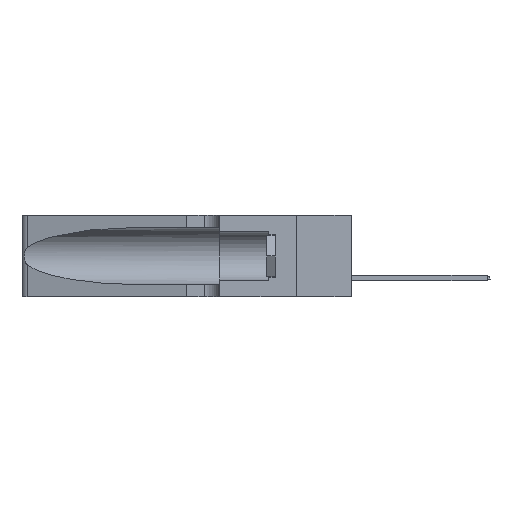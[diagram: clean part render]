
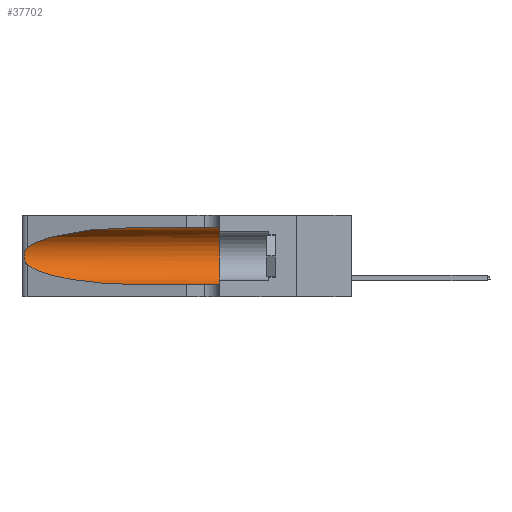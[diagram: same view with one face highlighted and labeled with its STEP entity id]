
A CAD part, left-side view. The second image highlights one B-rep face of the part: STEP entity #37702.
In plain terms, the highlighted cylindrical face has radius 3.308 mm (diameter 6.617 mm), a partial arc.
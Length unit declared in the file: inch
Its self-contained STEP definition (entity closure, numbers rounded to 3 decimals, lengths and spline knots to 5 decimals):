
#49 = EDGE_CURVE ( 'NONE', #26094, #20055, #33524, .T. ) ;
#1766 = ORIENTED_EDGE ( 'NONE', *, *, #3225, .T. ) ;
#2124 =( BOUNDED_CURVE ( )  B_SPLINE_CURVE ( 3, ( #13267, #25940, #29987, #39551 ),
 .UNSPECIFIED., .F., .F. ) 
 B_SPLINE_CURVE_WITH_KNOTS ( ( 4, 4 ),
 ( 3.44316, 4.71239 ),
 .UNSPECIFIED. ) 
 CURVE ( )  GEOMETRIC_REPRESENTATION_ITEM ( )  RATIONAL_B_SPLINE_CURVE ( ( 1., 0.87, 0.87, 1. ) ) 
 REPRESENTATION_ITEM ( '' )  );
#2389 = CARTESIAN_POINT ( 'NONE',  ( 0.26018, 1.23835, 0.19895 ) ) ;
#2554 = ORIENTED_EDGE ( 'NONE', *, *, #24998, .T. ) ;
#2798 = CARTESIAN_POINT ( 'NONE',  ( 0.25789, 1.23486, 0.15765 ) ) ;
#2854 = VECTOR ( 'NONE', #5763, 39.37008 ) ;
#3225 = EDGE_CURVE ( 'NONE', #15961, #3740, #2124, .T. ) ;
#3517 = AXIS2_PLACEMENT_3D ( 'NONE', #11135, #17967, #21017 ) ;
#3740 = VERTEX_POINT ( 'NONE', #24956 ) ;
#3848 = ORIENTED_EDGE ( 'NONE', *, *, #4998, .T. ) ;
#3862 = LINE ( 'NONE', #28295, #2854 ) ;
#4002 = CARTESIAN_POINT ( 'NONE',  ( 0.1305, 0.35, 0.05475 ) ) ;
#4131 = CYLINDRICAL_SURFACE ( 'NONE', #8900, 0.13025 ) ;
#4998 = EDGE_CURVE ( 'NONE', #3740, #20055, #3862, .T. ) ;
#5478 = CARTESIAN_POINT ( 'NONE',  ( 0.25787, 1.23484, 0.2124 ) ) ;
#5595 = CARTESIAN_POINT ( 'NONE',  ( 0.26075, 1.23896, 0.19203 ) ) ;
#5763 = DIRECTION ( 'NONE',  ( 0., -1., 0. ) ) ;
#6062 = DIRECTION ( 'NONE',  ( 0., -1., 0. ) ) ;
#8669 = CARTESIAN_POINT ( 'NONE',  ( 0.1305, 0.35, 0.31525 ) ) ;
#8900 = AXIS2_PLACEMENT_3D ( 'NONE', #13526, #38990, #19927 ) ;
#11135 = CARTESIAN_POINT ( 'NONE',  ( 0.1305, 0.35, 0.185 ) ) ;
#12410 = CARTESIAN_POINT ( 'NONE',  ( 0.25487, 1.22718, 0.22369 ) ) ;
#12671 = LINE ( 'NONE', #37898, #26615 ) ;
#13267 = CARTESIAN_POINT ( 'NONE',  ( 0.25487, 1.22718, 0.14631 ) ) ;
#13526 = CARTESIAN_POINT ( 'NONE',  ( 0.1305, 1.61858, 0.185 ) ) ;
#14025 = CARTESIAN_POINT ( 'NONE',  ( 0.2373, 1.15595, 0.28018 ) ) ;
#14151 = CARTESIAN_POINT ( 'NONE',  ( 0.1305, 0.72297, 0.31525 ) ) ;
#14511 = EDGE_CURVE ( 'NONE', #38973, #26094, #12671, .T. ) ;
#14899 = CARTESIAN_POINT ( 'NONE',  ( 0.25854, 1.2359, 0.20912 ) ) ;
#15696 = CARTESIAN_POINT ( 'NONE',  ( 0.25856, 1.23593, 0.16098 ) ) ;
#15961 = VERTEX_POINT ( 'NONE', #18734 ) ;
#17967 = DIRECTION ( 'NONE',  ( 0., 1., 0. ) ) ;
#18384 = CARTESIAN_POINT ( 'NONE',  ( 0.25555, 1.22994, 0.2215 ) ) ;
#18734 = CARTESIAN_POINT ( 'NONE',  ( 0.25487, 1.22718, 0.14631 ) ) ;
#19927 = DIRECTION ( 'NONE',  ( 0., 0., -1. ) ) ;
#20055 = VERTEX_POINT ( 'NONE', #4002 ) ;
#21017 = DIRECTION ( 'NONE',  ( 0., 0., 1. ) ) ;
#22402 = CARTESIAN_POINT ( 'NONE',  ( 0.25639, 1.23186, 0.15144 ) ) ;
#24956 = CARTESIAN_POINT ( 'NONE',  ( 0.1305, 0.72297, 0.05475 ) ) ;
#24998 = EDGE_CURVE ( 'NONE', #38973, #35078, #38556, .T. ) ;
#25572 = CARTESIAN_POINT ( 'NONE',  ( 0.25555, 1.22993, 0.14849 ) ) ;
#25646 = EDGE_LOOP ( 'NONE', ( #2554, #28320, #1766, #3848, #26276, #35158 ) ) ;
#25940 = CARTESIAN_POINT ( 'NONE',  ( 0.2373, 1.15595, 0.08982 ) ) ;
#26094 = VERTEX_POINT ( 'NONE', #8669 ) ;
#26276 = ORIENTED_EDGE ( 'NONE', *, *, #49, .F. ) ;
#26615 = VECTOR ( 'NONE', #6062, 39.37008 ) ;
#26858 = B_SPLINE_CURVE_WITH_KNOTS ( 'NONE', 3,
 ( #30785, #18384, #33970, #5478, #14899, #2389, #5595, #34247, #40623, #15696, #2798, #22402, #25572, #37967 ),
 .UNSPECIFIED., .F., .F.,
 ( 4, 2, 2, 2, 2, 2, 4 ),
 ( 0., 0.00027, 0.00053, 0.00107, 0.0016, 0.00187, 0.00214 ),
 .UNSPECIFIED. ) ;
#28295 = CARTESIAN_POINT ( 'NONE',  ( 0.1305, 1.61858, 0.05475 ) ) ;
#28320 = ORIENTED_EDGE ( 'NONE', *, *, #39826, .T. ) ;
#29987 = CARTESIAN_POINT ( 'NONE',  ( 0.18966, 0.96281, 0.05475 ) ) ;
#30785 = CARTESIAN_POINT ( 'NONE',  ( 0.25487, 1.22718, 0.22369 ) ) ;
#33469 = CARTESIAN_POINT ( 'NONE',  ( 0.1305, 0.72297, 0.31525 ) ) ;
#33509 = CARTESIAN_POINT ( 'NONE',  ( 0.25487, 1.22718, 0.22369 ) ) ;
#33524 = CIRCLE ( 'NONE', #3517, 0.13025 ) ;
#33970 = CARTESIAN_POINT ( 'NONE',  ( 0.25639, 1.23184, 0.21858 ) ) ;
#34247 = CARTESIAN_POINT ( 'NONE',  ( 0.26075, 1.23896, 0.178 ) ) ;
#35078 = VERTEX_POINT ( 'NONE', #12410 ) ;
#35158 = ORIENTED_EDGE ( 'NONE', *, *, #14511, .F. ) ;
#36305 = CARTESIAN_POINT ( 'NONE',  ( 0.18966, 0.96281, 0.31525 ) ) ;
#37702 = ADVANCED_FACE ( 'NONE', ( #39440 ), #4131, .F. ) ;
#37898 = CARTESIAN_POINT ( 'NONE',  ( 0.1305, 1.61858, 0.31525 ) ) ;
#37967 = CARTESIAN_POINT ( 'NONE',  ( 0.25487, 1.22718, 0.14631 ) ) ;
#38556 =( BOUNDED_CURVE ( )  B_SPLINE_CURVE ( 3, ( #14151, #36305, #14025, #33509 ),
 .UNSPECIFIED., .F., .F. ) 
 B_SPLINE_CURVE_WITH_KNOTS ( ( 4, 4 ),
 ( 1.5708, 2.84003 ),
 .UNSPECIFIED. ) 
 CURVE ( )  GEOMETRIC_REPRESENTATION_ITEM ( )  RATIONAL_B_SPLINE_CURVE ( ( 1., 0.87, 0.87, 1. ) ) 
 REPRESENTATION_ITEM ( '' )  );
#38973 = VERTEX_POINT ( 'NONE', #33469 ) ;
#38990 = DIRECTION ( 'NONE',  ( 0., -1., 0. ) ) ;
#39440 = FACE_OUTER_BOUND ( 'NONE', #25646, .T. ) ;
#39551 = CARTESIAN_POINT ( 'NONE',  ( 0.1305, 0.72297, 0.05475 ) ) ;
#39826 = EDGE_CURVE ( 'NONE', #35078, #15961, #26858, .T. ) ;
#40623 = CARTESIAN_POINT ( 'NONE',  ( 0.26017, 1.23833, 0.17102 ) ) ;
